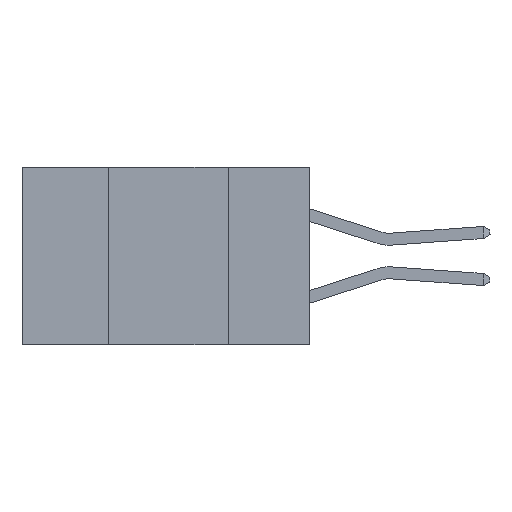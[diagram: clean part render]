
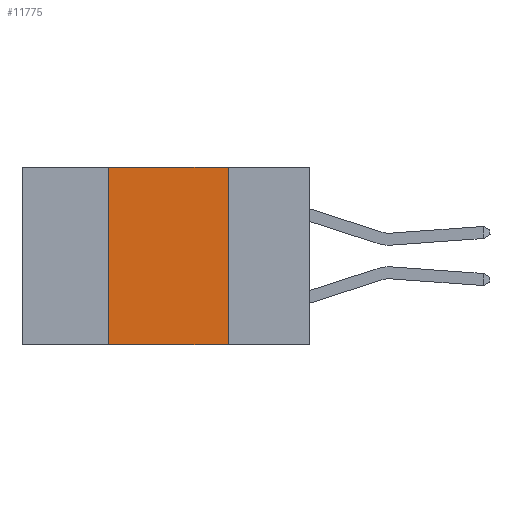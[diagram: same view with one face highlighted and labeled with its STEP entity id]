
A CAD part, left-side view. The second image highlights one B-rep face of the part: STEP entity #11775.
In plain terms, the highlighted planar face has unit normal (-1, 0, 0).
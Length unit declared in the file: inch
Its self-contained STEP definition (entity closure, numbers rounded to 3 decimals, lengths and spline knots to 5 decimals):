
#216 = AXIS2_PLACEMENT_3D ( 'NONE', #12698, #471, #15415 ) ;
#453 = EDGE_LOOP ( 'NONE', ( #13666, #5249, #15003, #8509 ) ) ;
#471 = DIRECTION ( 'NONE',  ( 1., 0., 0. ) ) ;
#1840 = CARTESIAN_POINT ( 'NONE',  ( 0., 0.17, -0.37 ) ) ;
#2061 = DIRECTION ( 'NONE',  ( 0., 0., -1. ) ) ;
#2652 = PLANE ( 'NONE',  #216 ) ;
#3474 = CARTESIAN_POINT ( 'NONE',  ( 0., 0.17, -0.37 ) ) ;
#4010 = DIRECTION ( 'NONE',  ( 0., -1., 0. ) ) ;
#4786 = VECTOR ( 'NONE', #4010, 39.37008 ) ;
#4929 = VERTEX_POINT ( 'NONE', #1840 ) ;
#5052 = DIRECTION ( 'NONE',  ( 0., -1., 0. ) ) ;
#5078 = VERTEX_POINT ( 'NONE', #9566 ) ;
#5102 = VECTOR ( 'NONE', #2061, 39.37008 ) ;
#5249 = ORIENTED_EDGE ( 'NONE', *, *, #7764, .F. ) ;
#5452 = CARTESIAN_POINT ( 'NONE',  ( 0., 0.17, 0. ) ) ;
#6604 = LINE ( 'NONE', #7661, #8376 ) ;
#7006 = LINE ( 'NONE', #3474, #5102 ) ;
#7661 = CARTESIAN_POINT ( 'NONE',  ( 0., 0.6, -0.37 ) ) ;
#7764 = EDGE_CURVE ( 'NONE', #5078, #8750, #15183, .T. ) ;
#8376 = VECTOR ( 'NONE', #5052, 39.37008 ) ;
#8509 = ORIENTED_EDGE ( 'NONE', *, *, #14884, .T. ) ;
#8750 = VERTEX_POINT ( 'NONE', #5452 ) ;
#8918 = CARTESIAN_POINT ( 'NONE',  ( 0., 0.42, -0.37 ) ) ;
#9165 = EDGE_CURVE ( 'NONE', #8750, #4929, #7006, .T. ) ;
#9187 = CARTESIAN_POINT ( 'NONE',  ( 0., 0.6, 0. ) ) ;
#9566 = CARTESIAN_POINT ( 'NONE',  ( 0., 0.42, 0. ) ) ;
#9816 = VECTOR ( 'NONE', #14045, 39.37008 ) ;
#10689 = VERTEX_POINT ( 'NONE', #13782 ) ;
#11323 = FACE_OUTER_BOUND ( 'NONE', #453, .T. ) ;
#11439 = EDGE_CURVE ( 'NONE', #10689, #5078, #13964, .T. ) ;
#11775 = ADVANCED_FACE ( 'NONE', ( #11323 ), #2652, .F. ) ;
#12698 = CARTESIAN_POINT ( 'NONE',  ( 0., 0.6, 0. ) ) ;
#13666 = ORIENTED_EDGE ( 'NONE', *, *, #9165, .F. ) ;
#13782 = CARTESIAN_POINT ( 'NONE',  ( 0., 0.42, -0.37 ) ) ;
#13964 = LINE ( 'NONE', #8918, #9816 ) ;
#14045 = DIRECTION ( 'NONE',  ( 0., 0., 1. ) ) ;
#14884 = EDGE_CURVE ( 'NONE', #10689, #4929, #6604, .T. ) ;
#15003 = ORIENTED_EDGE ( 'NONE', *, *, #11439, .F. ) ;
#15183 = LINE ( 'NONE', #9187, #4786 ) ;
#15415 = DIRECTION ( 'NONE',  ( 0., 0., -1. ) ) ;
